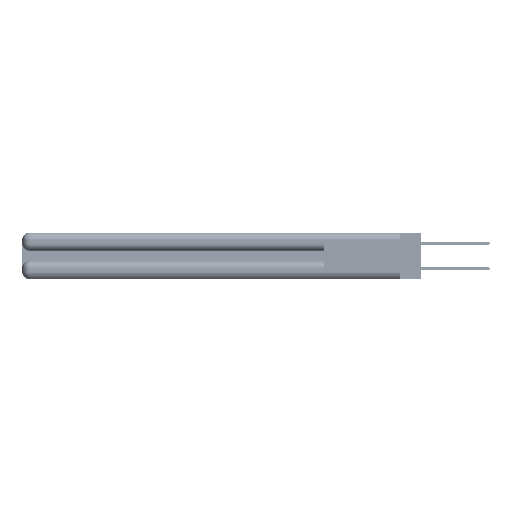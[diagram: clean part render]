
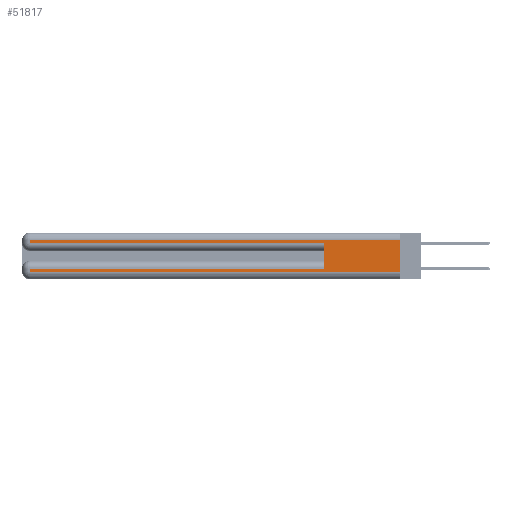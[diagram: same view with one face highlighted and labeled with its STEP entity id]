
A CAD part, left-side view. The second image highlights one B-rep face of the part: STEP entity #51817.
In plain terms, the highlighted planar face has unit normal (-1, 0, 0).
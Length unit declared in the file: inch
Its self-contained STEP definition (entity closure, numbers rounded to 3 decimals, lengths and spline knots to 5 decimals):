
#83 = ORIENTED_EDGE ( 'NONE', *, *, #12606, .F. ) ;
#663 = VECTOR ( 'NONE', #33106, 39.37008 ) ;
#683 = CARTESIAN_POINT ( 'NONE',  ( 0., 0., 0.31 ) ) ;
#1152 = VERTEX_POINT ( 'NONE', #33827 ) ;
#1290 = CARTESIAN_POINT ( 'NONE',  ( 0., 0., 0.06 ) ) ;
#2732 = ORIENTED_EDGE ( 'NONE', *, *, #39957, .T. ) ;
#3571 = EDGE_CURVE ( 'NONE', #5196, #23490, #14936, .T. ) ;
#5196 = VERTEX_POINT ( 'NONE', #16376 ) ;
#7503 = ORIENTED_EDGE ( 'NONE', *, *, #46269, .F. ) ;
#7943 = DIRECTION ( 'NONE',  ( 0., 0., -1. ) ) ;
#8217 = VERTEX_POINT ( 'NONE', #41765 ) ;
#10065 = LINE ( 'NONE', #40151, #51521 ) ;
#10863 = VERTEX_POINT ( 'NONE', #26573 ) ;
#11485 = DIRECTION ( 'NONE',  ( 0., 0., 1. ) ) ;
#11662 = CARTESIAN_POINT ( 'NONE',  ( 0., 0.6, 0.145 ) ) ;
#11771 = CARTESIAN_POINT ( 'NONE',  ( 0., 0.6, 0.285 ) ) ;
#11828 = CARTESIAN_POINT ( 'NONE',  ( 0., 0., 0.285 ) ) ;
#12606 = EDGE_CURVE ( 'NONE', #10863, #8217, #17156, .T. ) ;
#14936 = LINE ( 'NONE', #41114, #39417 ) ;
#16129 = ORIENTED_EDGE ( 'NONE', *, *, #31512, .T. ) ;
#16376 = CARTESIAN_POINT ( 'NONE',  ( 0., 0.6, 0.085 ) ) ;
#16701 = LINE ( 'NONE', #11662, #34329 ) ;
#16799 = CARTESIAN_POINT ( 'NONE',  ( 0., 2.94, 0.31 ) ) ;
#17156 = LINE ( 'NONE', #47266, #41052 ) ;
#17405 = DIRECTION ( 'NONE',  ( 0., 1., 0. ) ) ;
#17857 = CARTESIAN_POINT ( 'NONE',  ( 0., 2.94, 0.085 ) ) ;
#18243 = EDGE_CURVE ( 'NONE', #29191, #1152, #43665, .T. ) ;
#19638 = ORIENTED_EDGE ( 'NONE', *, *, #23854, .T. ) ;
#22732 = DIRECTION ( 'NONE',  ( 0., 0., -1. ) ) ;
#23490 = VERTEX_POINT ( 'NONE', #17857 ) ;
#23834 = VERTEX_POINT ( 'NONE', #40790 ) ;
#23854 = EDGE_CURVE ( 'NONE', #10863, #29191, #45842, .T. ) ;
#25131 = CARTESIAN_POINT ( 'NONE',  ( 0., 0., 0.37 ) ) ;
#25666 = DIRECTION ( 'NONE',  ( 0., -1., 0. ) ) ;
#26573 = CARTESIAN_POINT ( 'NONE',  ( 0., 0., 0.31 ) ) ;
#28649 = DIRECTION ( 'NONE',  ( 0., 0., -1. ) ) ;
#29191 = VERTEX_POINT ( 'NONE', #16799 ) ;
#31512 = EDGE_CURVE ( 'NONE', #1152, #32523, #50557, .T. ) ;
#31834 = DIRECTION ( 'NONE',  ( 0., -1., 0. ) ) ;
#32523 = VERTEX_POINT ( 'NONE', #11771 ) ;
#32875 = ORIENTED_EDGE ( 'NONE', *, *, #51884, .T. ) ;
#33106 = DIRECTION ( 'NONE',  ( 0., 1., 0. ) ) ;
#33827 = CARTESIAN_POINT ( 'NONE',  ( 0., 2.94, 0.285 ) ) ;
#34329 = VECTOR ( 'NONE', #11485, 39.37008 ) ;
#34393 = VECTOR ( 'NONE', #25666, 39.37008 ) ;
#36014 = CARTESIAN_POINT ( 'NONE',  ( 0., 2.94, 0.37 ) ) ;
#36521 = DIRECTION ( 'NONE',  ( 1., 0., 0. ) ) ;
#36697 = AXIS2_PLACEMENT_3D ( 'NONE', #25131, #36521, #28649 ) ;
#36903 = FACE_OUTER_BOUND ( 'NONE', #39086, .T. ) ;
#39086 = EDGE_LOOP ( 'NONE', ( #83, #19638, #46052, #16129, #7503, #41993, #2732, #32875 ) ) ;
#39417 = VECTOR ( 'NONE', #17405, 39.37008 ) ;
#39957 = EDGE_CURVE ( 'NONE', #23490, #23834, #10065, .T. ) ;
#40151 = CARTESIAN_POINT ( 'NONE',  ( 0., 2.94, 0.37 ) ) ;
#40790 = CARTESIAN_POINT ( 'NONE',  ( 0., 2.94, 0.06 ) ) ;
#41052 = VECTOR ( 'NONE', #22732, 39.37008 ) ;
#41114 = CARTESIAN_POINT ( 'NONE',  ( 0., 0., 0.085 ) ) ;
#41765 = CARTESIAN_POINT ( 'NONE',  ( 0., 0., 0.06 ) ) ;
#41993 = ORIENTED_EDGE ( 'NONE', *, *, #3571, .T. ) ;
#43665 = LINE ( 'NONE', #36014, #44268 ) ;
#44268 = VECTOR ( 'NONE', #7943, 39.37008 ) ;
#45842 = LINE ( 'NONE', #683, #663 ) ;
#46052 = ORIENTED_EDGE ( 'NONE', *, *, #18243, .T. ) ;
#46269 = EDGE_CURVE ( 'NONE', #5196, #32523, #16701, .T. ) ;
#47266 = CARTESIAN_POINT ( 'NONE',  ( 0., 0., 0.37 ) ) ;
#48617 = VECTOR ( 'NONE', #31834, 39.37008 ) ;
#48813 = LINE ( 'NONE', #1290, #34393 ) ;
#49144 = PLANE ( 'NONE',  #36697 ) ;
#50557 = LINE ( 'NONE', #11828, #48617 ) ;
#51521 = VECTOR ( 'NONE', #51950, 39.37008 ) ;
#51817 = ADVANCED_FACE ( 'NONE', ( #36903 ), #49144, .F. ) ;
#51884 = EDGE_CURVE ( 'NONE', #23834, #8217, #48813, .T. ) ;
#51950 = DIRECTION ( 'NONE',  ( 0., 0., -1. ) ) ;
